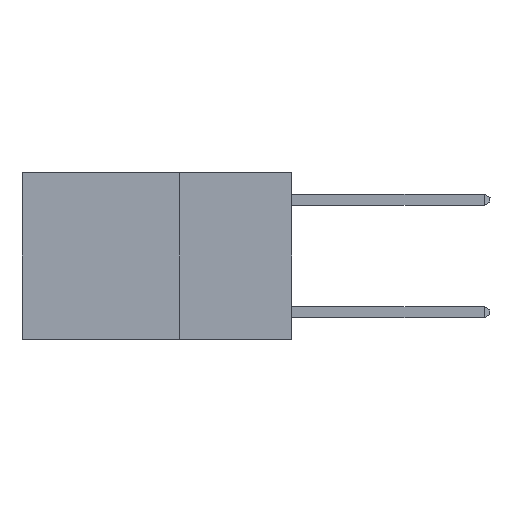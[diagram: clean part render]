
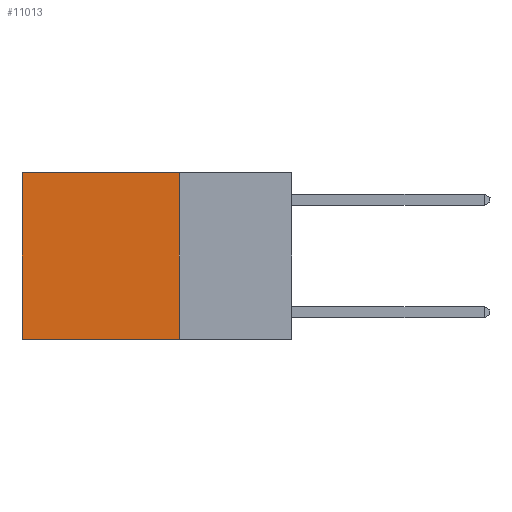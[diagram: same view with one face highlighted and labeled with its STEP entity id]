
A CAD part, left-side view. The second image highlights one B-rep face of the part: STEP entity #11013.
In plain terms, the highlighted planar face has unit normal (-1, 0, 0).
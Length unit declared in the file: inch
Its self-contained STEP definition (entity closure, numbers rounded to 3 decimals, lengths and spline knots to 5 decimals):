
#139 = VECTOR ( 'NONE', #10155, 39.37008 ) ;
#367 = CARTESIAN_POINT ( 'NONE',  ( 0.2625, 0.6, 0. ) ) ;
#685 = VERTEX_POINT ( 'NONE', #367 ) ;
#1122 = CARTESIAN_POINT ( 'NONE',  ( 0.2625, 0.25, 0. ) ) ;
#1393 = VECTOR ( 'NONE', #1822, 39.37008 ) ;
#1822 = DIRECTION ( 'NONE',  ( 0., 0., -1. ) ) ;
#2997 = CARTESIAN_POINT ( 'NONE',  ( 0.2625, 0.25, -0.37 ) ) ;
#3186 = EDGE_CURVE ( 'NONE', #13731, #14400, #11124, .T. ) ;
#3326 = VERTEX_POINT ( 'NONE', #3875 ) ;
#3875 = CARTESIAN_POINT ( 'NONE',  ( 0.2625, 0.6, -0.37 ) ) ;
#3934 = EDGE_CURVE ( 'NONE', #13731, #685, #9930, .T. ) ;
#5097 = ORIENTED_EDGE ( 'NONE', *, *, #8961, .F. ) ;
#5162 = ORIENTED_EDGE ( 'NONE', *, *, #10299, .T. ) ;
#7083 = ORIENTED_EDGE ( 'NONE', *, *, #3186, .F. ) ;
#7851 = LINE ( 'NONE', #12461, #8951 ) ;
#8104 = DIRECTION ( 'NONE',  ( 0., 1., 0. ) ) ;
#8440 = EDGE_LOOP ( 'NONE', ( #5162, #5097, #7083, #10221 ) ) ;
#8951 = VECTOR ( 'NONE', #9228, 39.37008 ) ;
#8961 = EDGE_CURVE ( 'NONE', #14400, #3326, #12846, .T. ) ;
#9228 = DIRECTION ( 'NONE',  ( 0., 0., -1. ) ) ;
#9930 = LINE ( 'NONE', #13482, #139 ) ;
#10155 = DIRECTION ( 'NONE',  ( 0., 1., 0. ) ) ;
#10214 = CARTESIAN_POINT ( 'NONE',  ( 0.2625, 0.25, -0.37 ) ) ;
#10221 = ORIENTED_EDGE ( 'NONE', *, *, #3934, .T. ) ;
#10299 = EDGE_CURVE ( 'NONE', #685, #3326, #7851, .T. ) ;
#10553 = DIRECTION ( 'NONE',  ( 1., 0., 0. ) ) ;
#11013 = ADVANCED_FACE ( 'NONE', ( #11541 ), #12733, .F. ) ;
#11124 = LINE ( 'NONE', #12250, #1393 ) ;
#11490 = VECTOR ( 'NONE', #8104, 39.37008 ) ;
#11541 = FACE_OUTER_BOUND ( 'NONE', #8440, .T. ) ;
#12250 = CARTESIAN_POINT ( 'NONE',  ( 0.2625, 0.25, 0. ) ) ;
#12461 = CARTESIAN_POINT ( 'NONE',  ( 0.2625, 0.6, 0. ) ) ;
#12609 = AXIS2_PLACEMENT_3D ( 'NONE', #1122, #10553, #12880 ) ;
#12733 = PLANE ( 'NONE',  #12609 ) ;
#12846 = LINE ( 'NONE', #10214, #11490 ) ;
#12880 = DIRECTION ( 'NONE',  ( 0., 0., -1. ) ) ;
#13482 = CARTESIAN_POINT ( 'NONE',  ( 0.2625, 0.25, 0. ) ) ;
#13731 = VERTEX_POINT ( 'NONE', #14258 ) ;
#14258 = CARTESIAN_POINT ( 'NONE',  ( 0.2625, 0.25, 0. ) ) ;
#14400 = VERTEX_POINT ( 'NONE', #2997 ) ;
